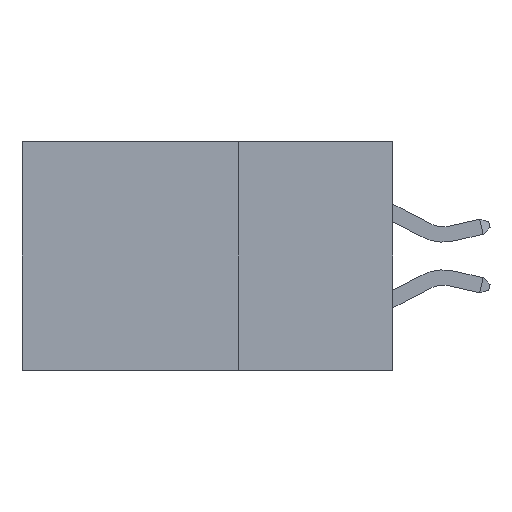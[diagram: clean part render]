
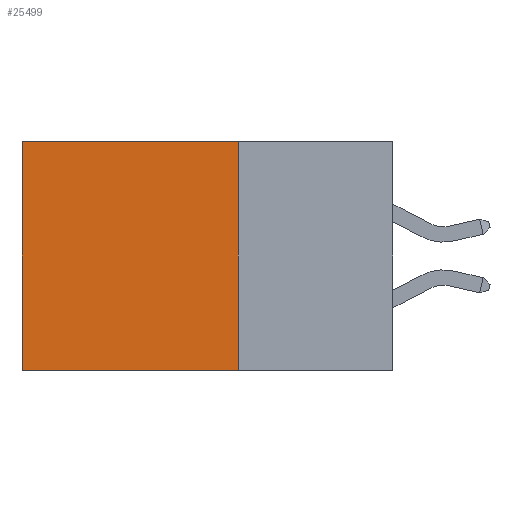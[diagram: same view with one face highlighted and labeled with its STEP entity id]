
A CAD part, left-side view. The second image highlights one B-rep face of the part: STEP entity #25499.
In plain terms, the highlighted planar face has unit normal (-1, 0, 0).
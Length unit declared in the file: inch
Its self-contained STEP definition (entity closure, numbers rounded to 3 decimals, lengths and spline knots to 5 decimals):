
#64 = EDGE_CURVE ( 'NONE', #16036, #12239, #27812, .T. ) ;
#119 = LINE ( 'NONE', #30806, #6527 ) ;
#987 = FACE_OUTER_BOUND ( 'NONE', #9972, .T. ) ;
#1297 = EDGE_CURVE ( 'NONE', #11340, #12239, #7564, .T. ) ;
#2831 = DIRECTION ( 'NONE',  ( 0., 1., 0. ) ) ;
#3187 = ORIENTED_EDGE ( 'NONE', *, *, #1297, .T. ) ;
#3362 = ORIENTED_EDGE ( 'NONE', *, *, #20219, .F. ) ;
#3446 = LINE ( 'NONE', #20657, #23940 ) ;
#3485 = AXIS2_PLACEMENT_3D ( 'NONE', #9881, #17323, #17533 ) ;
#4983 = CARTESIAN_POINT ( 'NONE',  ( 0.2875, 0.6, -0.37 ) ) ;
#5227 = DIRECTION ( 'NONE',  ( 0., 0., -1. ) ) ;
#5560 = VERTEX_POINT ( 'NONE', #25781 ) ;
#6527 = VECTOR ( 'NONE', #5227, 39.37008 ) ;
#7530 = CARTESIAN_POINT ( 'NONE',  ( 0.2875, 0.25, -0.37 ) ) ;
#7564 = LINE ( 'NONE', #32707, #17624 ) ;
#9881 = CARTESIAN_POINT ( 'NONE',  ( 0.2875, 0.25, 0. ) ) ;
#9972 = EDGE_LOOP ( 'NONE', ( #3187, #13850, #3362, #15917 ) ) ;
#11001 = CARTESIAN_POINT ( 'NONE',  ( 0.2875, 0.25, -0.37 ) ) ;
#11340 = VERTEX_POINT ( 'NONE', #18298 ) ;
#12239 = VERTEX_POINT ( 'NONE', #4983 ) ;
#13850 = ORIENTED_EDGE ( 'NONE', *, *, #64, .F. ) ;
#15917 = ORIENTED_EDGE ( 'NONE', *, *, #24476, .T. ) ;
#16036 = VERTEX_POINT ( 'NONE', #11001 ) ;
#16663 = DIRECTION ( 'NONE',  ( 0., 1., 0. ) ) ;
#17323 = DIRECTION ( 'NONE',  ( 1., 0., 0. ) ) ;
#17533 = DIRECTION ( 'NONE',  ( 0., 0., -1. ) ) ;
#17624 = VECTOR ( 'NONE', #22387, 39.37008 ) ;
#18298 = CARTESIAN_POINT ( 'NONE',  ( 0.2875, 0.6, 0. ) ) ;
#19325 = VECTOR ( 'NONE', #16663, 39.37008 ) ;
#20219 = EDGE_CURVE ( 'NONE', #5560, #16036, #119, .T. ) ;
#20657 = CARTESIAN_POINT ( 'NONE',  ( 0.2875, 0.25, 0. ) ) ;
#22387 = DIRECTION ( 'NONE',  ( 0., 0., -1. ) ) ;
#23940 = VECTOR ( 'NONE', #2831, 39.37008 ) ;
#24476 = EDGE_CURVE ( 'NONE', #5560, #11340, #3446, .T. ) ;
#25189 = PLANE ( 'NONE',  #3485 ) ;
#25499 = ADVANCED_FACE ( 'NONE', ( #987 ), #25189, .F. ) ;
#25781 = CARTESIAN_POINT ( 'NONE',  ( 0.2875, 0.25, 0. ) ) ;
#27812 = LINE ( 'NONE', #7530, #19325 ) ;
#30806 = CARTESIAN_POINT ( 'NONE',  ( 0.2875, 0.25, 0. ) ) ;
#32707 = CARTESIAN_POINT ( 'NONE',  ( 0.2875, 0.6, 0. ) ) ;
